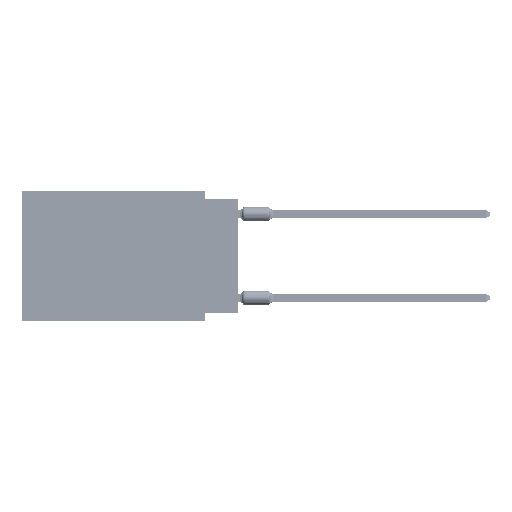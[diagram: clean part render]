
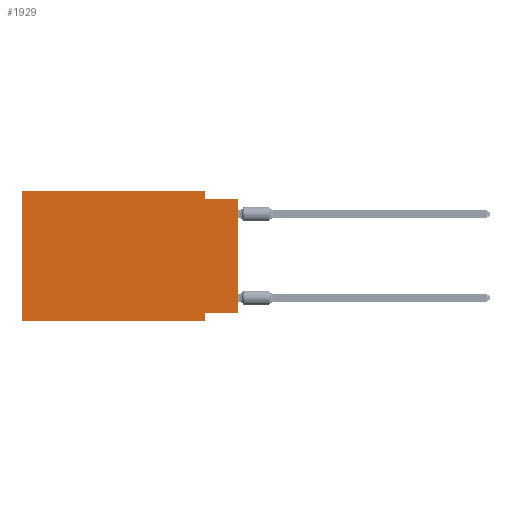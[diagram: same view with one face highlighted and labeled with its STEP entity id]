
A CAD part, left-side view. The second image highlights one B-rep face of the part: STEP entity #1929.
In plain terms, the highlighted planar face has unit normal (-1, 0, 0).
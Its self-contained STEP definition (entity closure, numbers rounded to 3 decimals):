
#676 = LINE ( 'NONE', #39933, #33229 ) ;
#1606 = DIRECTION ( 'NONE',  ( 0., 0., -1. ) ) ;
#1929 = ADVANCED_FACE ( 'NONE', ( #3068 ), #64577, .F. ) ;
#2441 = CARTESIAN_POINT ( 'NONE',  ( 0., 16.383, 0. ) ) ;
#2747 = EDGE_CURVE ( 'NONE', #29083, #4509, #7621, .T. ) ;
#2783 = LINE ( 'NONE', #60205, #67318 ) ;
#3068 = FACE_OUTER_BOUND ( 'NONE', #18577, .T. ) ;
#3895 = VERTEX_POINT ( 'NONE', #67470 ) ;
#4270 = DIRECTION ( 'NONE',  ( 0., 0., -1. ) ) ;
#4509 = VERTEX_POINT ( 'NONE', #48297 ) ;
#5479 = CARTESIAN_POINT ( 'NONE',  ( 0., 2.54, -9.906 ) ) ;
#7621 = LINE ( 'NONE', #2441, #40520 ) ;
#9942 = DIRECTION ( 'NONE',  ( 0., 1., 0. ) ) ;
#13265 = EDGE_CURVE ( 'NONE', #4509, #3895, #31547, .T. ) ;
#14236 = ORIENTED_EDGE ( 'NONE', *, *, #14453, .T. ) ;
#14253 = DIRECTION ( 'NONE',  ( 0., 0., 1. ) ) ;
#14453 = EDGE_CURVE ( 'NONE', #71310, #24950, #2783, .T. ) ;
#15139 = VECTOR ( 'NONE', #65660, 1000. ) ;
#16706 = EDGE_CURVE ( 'NONE', #3895, #24950, #676, .T. ) ;
#17042 = CARTESIAN_POINT ( 'NONE',  ( 0., 0., -0.635 ) ) ;
#17606 = ORIENTED_EDGE ( 'NONE', *, *, #35026, .F. ) ;
#18577 = EDGE_LOOP ( 'NONE', ( #14236, #60095, #43534, #22459, #70621, #42325, #17606, #60457 ) ) ;
#20419 = CARTESIAN_POINT ( 'NONE',  ( 0., 2.54, 0. ) ) ;
#22459 = ORIENTED_EDGE ( 'NONE', *, *, #2747, .F. ) ;
#24950 = VERTEX_POINT ( 'NONE', #17042 ) ;
#28321 = VERTEX_POINT ( 'NONE', #32909 ) ;
#28380 = EDGE_CURVE ( 'NONE', #71310, #28321, #44016, .T. ) ;
#28999 = VECTOR ( 'NONE', #41620, 1000. ) ;
#29083 = VERTEX_POINT ( 'NONE', #68741 ) ;
#30204 = VECTOR ( 'NONE', #9942, 1000. ) ;
#31146 = EDGE_CURVE ( 'NONE', #35666, #71975, #70524, .T. ) ;
#31547 = LINE ( 'NONE', #20419, #15139 ) ;
#31602 = CARTESIAN_POINT ( 'NONE',  ( 0., 16.383, -9.906 ) ) ;
#32909 = CARTESIAN_POINT ( 'NONE',  ( 0., 2.54, -9.271 ) ) ;
#33229 = VECTOR ( 'NONE', #39570, 1000. ) ;
#35026 = EDGE_CURVE ( 'NONE', #28321, #71975, #44264, .T. ) ;
#35666 = VERTEX_POINT ( 'NONE', #53387 ) ;
#37238 = CARTESIAN_POINT ( 'NONE',  ( 0., 2.54, -9.906 ) ) ;
#38462 = CARTESIAN_POINT ( 'NONE',  ( 0., 0., -9.271 ) ) ;
#39570 = DIRECTION ( 'NONE',  ( 0., -1., 0. ) ) ;
#39933 = CARTESIAN_POINT ( 'NONE',  ( 0., 0., -0.635 ) ) ;
#40520 = VECTOR ( 'NONE', #63955, 1000. ) ;
#41620 = DIRECTION ( 'NONE',  ( 0., -1., 0. ) ) ;
#41952 = DIRECTION ( 'NONE',  ( 1., 0., 0. ) ) ;
#42325 = ORIENTED_EDGE ( 'NONE', *, *, #31146, .T. ) ;
#43534 = ORIENTED_EDGE ( 'NONE', *, *, #13265, .F. ) ;
#43812 = VECTOR ( 'NONE', #69468, 1000. ) ;
#44016 = LINE ( 'NONE', #38462, #30204 ) ;
#44264 = LINE ( 'NONE', #37238, #67117 ) ;
#48297 = CARTESIAN_POINT ( 'NONE',  ( 0., 2.54, 0. ) ) ;
#49910 = EDGE_CURVE ( 'NONE', #35666, #29083, #69102, .T. ) ;
#53387 = CARTESIAN_POINT ( 'NONE',  ( 0., 16.383, -9.906 ) ) ;
#56502 = CARTESIAN_POINT ( 'NONE',  ( 0., 0., -9.271 ) ) ;
#57611 = CARTESIAN_POINT ( 'NONE',  ( 0., 16.383, 0. ) ) ;
#60095 = ORIENTED_EDGE ( 'NONE', *, *, #16706, .F. ) ;
#60205 = CARTESIAN_POINT ( 'NONE',  ( 0., 0., 0. ) ) ;
#60457 = ORIENTED_EDGE ( 'NONE', *, *, #28380, .F. ) ;
#62927 = AXIS2_PLACEMENT_3D ( 'NONE', #70496, #41952, #1606 ) ;
#63955 = DIRECTION ( 'NONE',  ( 0., -1., 0. ) ) ;
#64577 = PLANE ( 'NONE',  #62927 ) ;
#65660 = DIRECTION ( 'NONE',  ( 0., 0., -1. ) ) ;
#67117 = VECTOR ( 'NONE', #4270, 1000. ) ;
#67318 = VECTOR ( 'NONE', #14253, 1000. ) ;
#67470 = CARTESIAN_POINT ( 'NONE',  ( 0., 2.54, -0.635 ) ) ;
#68741 = CARTESIAN_POINT ( 'NONE',  ( 0., 16.383, 0. ) ) ;
#69102 = LINE ( 'NONE', #57611, #43812 ) ;
#69468 = DIRECTION ( 'NONE',  ( 0., 0., 1. ) ) ;
#70496 = CARTESIAN_POINT ( 'NONE',  ( 0., 16.383, 0. ) ) ;
#70524 = LINE ( 'NONE', #31602, #28999 ) ;
#70621 = ORIENTED_EDGE ( 'NONE', *, *, #49910, .F. ) ;
#71310 = VERTEX_POINT ( 'NONE', #56502 ) ;
#71975 = VERTEX_POINT ( 'NONE', #5479 ) ;
